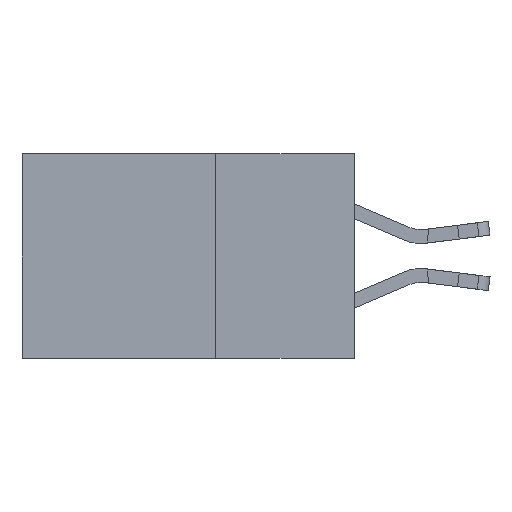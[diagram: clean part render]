
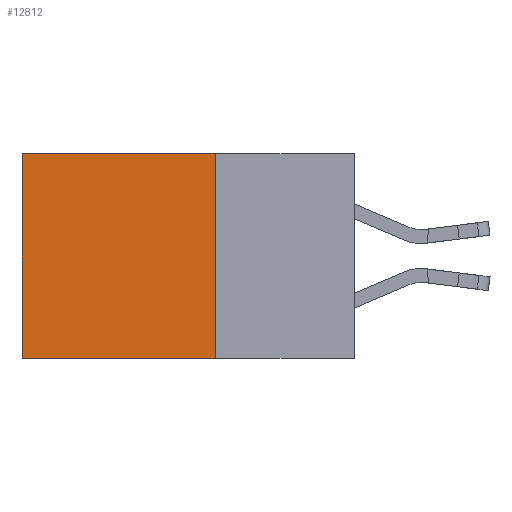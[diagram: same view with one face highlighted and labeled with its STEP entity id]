
A CAD part, left-side view. The second image highlights one B-rep face of the part: STEP entity #12812.
In plain terms, the highlighted planar face has unit normal (-1, 0, 0).
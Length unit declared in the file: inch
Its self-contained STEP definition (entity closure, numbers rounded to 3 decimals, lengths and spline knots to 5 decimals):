
#37 = VERTEX_POINT ( 'NONE', #5770 ) ;
#2022 = ORIENTED_EDGE ( 'NONE', *, *, #6759, .F. ) ;
#2397 = EDGE_LOOP ( 'NONE', ( #10911, #3807, #2022, #11201 ) ) ;
#2570 = DIRECTION ( 'NONE',  ( 0., 1., 0. ) ) ;
#3347 = CARTESIAN_POINT ( 'NONE',  ( 0.2615, 0.25, -0.37 ) ) ;
#3680 = VERTEX_POINT ( 'NONE', #7060 ) ;
#3702 = EDGE_CURVE ( 'NONE', #37, #3680, #7113, .T. ) ;
#3727 = AXIS2_PLACEMENT_3D ( 'NONE', #3347, #12828, #6593 ) ;
#3807 = ORIENTED_EDGE ( 'NONE', *, *, #3702, .F. ) ;
#3847 = LINE ( 'NONE', #8587, #11997 ) ;
#4083 = DIRECTION ( 'NONE',  ( 0., 1., 0. ) ) ;
#4227 = VECTOR ( 'NONE', #8164, 39.37008 ) ;
#4251 = VECTOR ( 'NONE', #4083, 39.37008 ) ;
#5334 = EDGE_CURVE ( 'NONE', #11500, #3680, #9933, .T. ) ;
#5515 = PLANE ( 'NONE',  #3727 ) ;
#5770 = CARTESIAN_POINT ( 'NONE',  ( 0.2615, 0.25, -0.37 ) ) ;
#5888 = CARTESIAN_POINT ( 'NONE',  ( 0.2615, 0.25, 0. ) ) ;
#6421 = VERTEX_POINT ( 'NONE', #12440 ) ;
#6529 = CARTESIAN_POINT ( 'NONE',  ( 0.2615, 0.6, 0. ) ) ;
#6536 = CARTESIAN_POINT ( 'NONE',  ( 0.2615, 0.25, -0.37 ) ) ;
#6593 = DIRECTION ( 'NONE',  ( 0., 0., -1. ) ) ;
#6759 = EDGE_CURVE ( 'NONE', #6421, #37, #3847, .T. ) ;
#7060 = CARTESIAN_POINT ( 'NONE',  ( 0.2615, 0.6, -0.37 ) ) ;
#7113 = LINE ( 'NONE', #6536, #4251 ) ;
#8029 = CARTESIAN_POINT ( 'NONE',  ( 0.2615, 0.6, -0.37 ) ) ;
#8164 = DIRECTION ( 'NONE',  ( 0., 0., -1. ) ) ;
#8587 = CARTESIAN_POINT ( 'NONE',  ( 0.2615, 0.25, -0.37 ) ) ;
#8639 = EDGE_CURVE ( 'NONE', #6421, #11500, #11945, .T. ) ;
#9046 = DIRECTION ( 'NONE',  ( 0., 0., -1. ) ) ;
#9334 = FACE_OUTER_BOUND ( 'NONE', #2397, .T. ) ;
#9500 = VECTOR ( 'NONE', #2570, 39.37008 ) ;
#9933 = LINE ( 'NONE', #8029, #4227 ) ;
#10911 = ORIENTED_EDGE ( 'NONE', *, *, #5334, .T. ) ;
#11201 = ORIENTED_EDGE ( 'NONE', *, *, #8639, .T. ) ;
#11500 = VERTEX_POINT ( 'NONE', #6529 ) ;
#11945 = LINE ( 'NONE', #5888, #9500 ) ;
#11997 = VECTOR ( 'NONE', #9046, 39.37008 ) ;
#12440 = CARTESIAN_POINT ( 'NONE',  ( 0.2615, 0.25, 0. ) ) ;
#12812 = ADVANCED_FACE ( 'NONE', ( #9334 ), #5515, .F. ) ;
#12828 = DIRECTION ( 'NONE',  ( 1., 0., 0. ) ) ;
